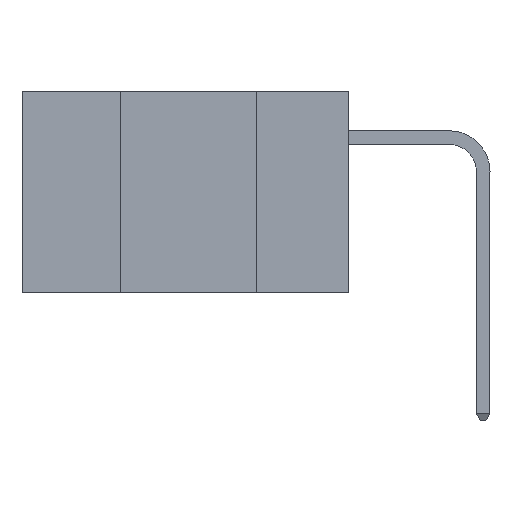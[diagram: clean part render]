
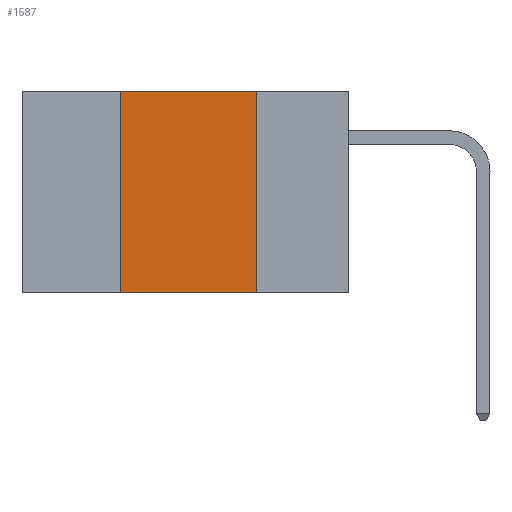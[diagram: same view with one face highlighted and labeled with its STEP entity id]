
A CAD part, left-side view. The second image highlights one B-rep face of the part: STEP entity #1587.
In plain terms, the highlighted planar face has unit normal (-1, 0, 0).
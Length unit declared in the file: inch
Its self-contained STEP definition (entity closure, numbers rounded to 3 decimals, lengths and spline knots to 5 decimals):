
#334 = CARTESIAN_POINT ( 'NONE',  ( 0., 0.6, 0. ) ) ;
#455 = LINE ( 'NONE', #334, #4064 ) ;
#629 = CARTESIAN_POINT ( 'NONE',  ( 0., 0.6, 0. ) ) ;
#1565 = EDGE_CURVE ( 'NONE', #18164, #14675, #15857, .T. ) ;
#1587 = ADVANCED_FACE ( 'NONE', ( #3814 ), #15625, .F. ) ;
#1889 = DIRECTION ( 'NONE',  ( 0., -1., 0. ) ) ;
#1969 = LINE ( 'NONE', #4654, #17063 ) ;
#3737 = DIRECTION ( 'NONE',  ( 0., -1., 0. ) ) ;
#3814 = FACE_OUTER_BOUND ( 'NONE', #9325, .T. ) ;
#4064 = VECTOR ( 'NONE', #1889, 39.37008 ) ;
#4110 = EDGE_CURVE ( 'NONE', #7787, #14675, #1969, .T. ) ;
#4654 = CARTESIAN_POINT ( 'NONE',  ( 0., 0.17, 0. ) ) ;
#4846 = DIRECTION ( 'NONE',  ( 0., 0., -1. ) ) ;
#5517 = EDGE_CURVE ( 'NONE', #10917, #7787, #455, .T. ) ;
#6092 = CARTESIAN_POINT ( 'NONE',  ( 0., 0.6, -0.37 ) ) ;
#7047 = ORIENTED_EDGE ( 'NONE', *, *, #4110, .F. ) ;
#7787 = VERTEX_POINT ( 'NONE', #19462 ) ;
#7903 = VECTOR ( 'NONE', #3737, 39.37008 ) ;
#8235 = CARTESIAN_POINT ( 'NONE',  ( 0., 0.42, 0. ) ) ;
#9325 = EDGE_LOOP ( 'NONE', ( #7047, #12782, #12561, #14971 ) ) ;
#9482 = CARTESIAN_POINT ( 'NONE',  ( 0., 0.17, -0.37 ) ) ;
#10599 = LINE ( 'NONE', #11106, #14589 ) ;
#10917 = VERTEX_POINT ( 'NONE', #8235 ) ;
#11106 = CARTESIAN_POINT ( 'NONE',  ( 0., 0.42, 0. ) ) ;
#11140 = DIRECTION ( 'NONE',  ( 0., 0., -1. ) ) ;
#12561 = ORIENTED_EDGE ( 'NONE', *, *, #17961, .F. ) ;
#12634 = DIRECTION ( 'NONE',  ( 0., 0., 1. ) ) ;
#12782 = ORIENTED_EDGE ( 'NONE', *, *, #5517, .F. ) ;
#12999 = AXIS2_PLACEMENT_3D ( 'NONE', #629, #18529, #11140 ) ;
#14589 = VECTOR ( 'NONE', #12634, 39.37008 ) ;
#14675 = VERTEX_POINT ( 'NONE', #9482 ) ;
#14971 = ORIENTED_EDGE ( 'NONE', *, *, #1565, .T. ) ;
#15625 = PLANE ( 'NONE',  #12999 ) ;
#15857 = LINE ( 'NONE', #6092, #7903 ) ;
#16143 = CARTESIAN_POINT ( 'NONE',  ( 0., 0.42, -0.37 ) ) ;
#17063 = VECTOR ( 'NONE', #4846, 39.37008 ) ;
#17961 = EDGE_CURVE ( 'NONE', #18164, #10917, #10599, .T. ) ;
#18164 = VERTEX_POINT ( 'NONE', #16143 ) ;
#18529 = DIRECTION ( 'NONE',  ( 1., 0., 0. ) ) ;
#19462 = CARTESIAN_POINT ( 'NONE',  ( 0., 0.17, 0. ) ) ;
